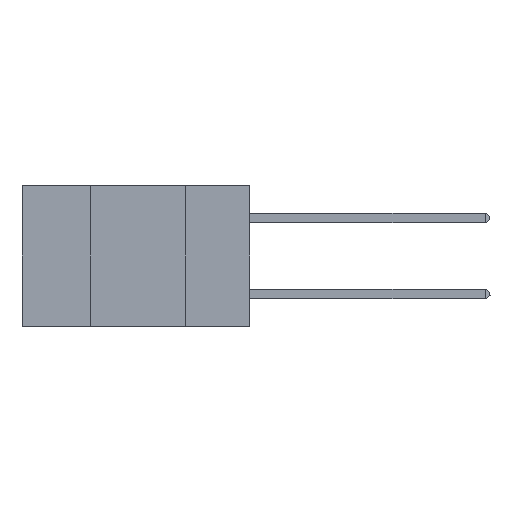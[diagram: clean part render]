
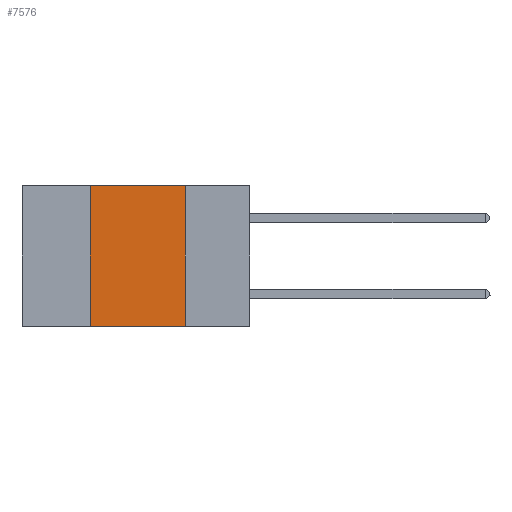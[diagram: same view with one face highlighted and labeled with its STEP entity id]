
A CAD part, left-side view. The second image highlights one B-rep face of the part: STEP entity #7576.
In plain terms, the highlighted planar face has unit normal (-1, 0, 0).
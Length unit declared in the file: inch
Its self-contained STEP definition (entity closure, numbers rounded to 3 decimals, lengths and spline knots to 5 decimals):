
#2159 = DIRECTION ( 'NONE',  ( 0., 0., -1. ) ) ;
#3424 = VERTEX_POINT ( 'NONE', #4639 ) ;
#3954 = LINE ( 'NONE', #19360, #35943 ) ;
#4639 = CARTESIAN_POINT ( 'NONE',  ( 0., 0.17, 0. ) ) ;
#5986 = PLANE ( 'NONE',  #19285 ) ;
#7493 = CARTESIAN_POINT ( 'NONE',  ( 0., 0.17, -0.37 ) ) ;
#7576 = ADVANCED_FACE ( 'NONE', ( #30257 ), #5986, .F. ) ;
#7616 = EDGE_CURVE ( 'NONE', #24308, #36872, #15076, .T. ) ;
#8046 = CARTESIAN_POINT ( 'NONE',  ( 0., 0.42, -0.37 ) ) ;
#8691 = LINE ( 'NONE', #20282, #34585 ) ;
#8799 = ORIENTED_EDGE ( 'NONE', *, *, #32287, .F. ) ;
#9283 = EDGE_CURVE ( 'NONE', #36872, #3424, #35836, .T. ) ;
#9298 = VERTEX_POINT ( 'NONE', #7493 ) ;
#9438 = CARTESIAN_POINT ( 'NONE',  ( 0., 0.6, 0. ) ) ;
#13134 = EDGE_CURVE ( 'NONE', #24308, #9298, #8691, .T. ) ;
#13432 = ORIENTED_EDGE ( 'NONE', *, *, #9283, .F. ) ;
#14220 = VECTOR ( 'NONE', #29883, 39.37008 ) ;
#15076 = LINE ( 'NONE', #32765, #14220 ) ;
#15848 = ORIENTED_EDGE ( 'NONE', *, *, #13134, .T. ) ;
#18309 = DIRECTION ( 'NONE',  ( 0., -1., 0. ) ) ;
#19285 = AXIS2_PLACEMENT_3D ( 'NONE', #24116, #35853, #35283 ) ;
#19360 = CARTESIAN_POINT ( 'NONE',  ( 0., 0.17, 0. ) ) ;
#20282 = CARTESIAN_POINT ( 'NONE',  ( 0., 0.6, -0.37 ) ) ;
#20360 = ORIENTED_EDGE ( 'NONE', *, *, #7616, .F. ) ;
#20687 = EDGE_LOOP ( 'NONE', ( #8799, #13432, #20360, #15848 ) ) ;
#22156 = VECTOR ( 'NONE', #18309, 39.37008 ) ;
#24116 = CARTESIAN_POINT ( 'NONE',  ( 0., 0.6, 0. ) ) ;
#24308 = VERTEX_POINT ( 'NONE', #8046 ) ;
#27522 = CARTESIAN_POINT ( 'NONE',  ( 0., 0.42, 0. ) ) ;
#29883 = DIRECTION ( 'NONE',  ( 0., 0., 1. ) ) ;
#30257 = FACE_OUTER_BOUND ( 'NONE', #20687, .T. ) ;
#32287 = EDGE_CURVE ( 'NONE', #3424, #9298, #3954, .T. ) ;
#32765 = CARTESIAN_POINT ( 'NONE',  ( 0., 0.42, 0. ) ) ;
#34585 = VECTOR ( 'NONE', #35652, 39.37008 ) ;
#35283 = DIRECTION ( 'NONE',  ( 0., 0., -1. ) ) ;
#35652 = DIRECTION ( 'NONE',  ( 0., -1., 0. ) ) ;
#35836 = LINE ( 'NONE', #9438, #22156 ) ;
#35853 = DIRECTION ( 'NONE',  ( 1., 0., 0. ) ) ;
#35943 = VECTOR ( 'NONE', #2159, 39.37008 ) ;
#36872 = VERTEX_POINT ( 'NONE', #27522 ) ;
